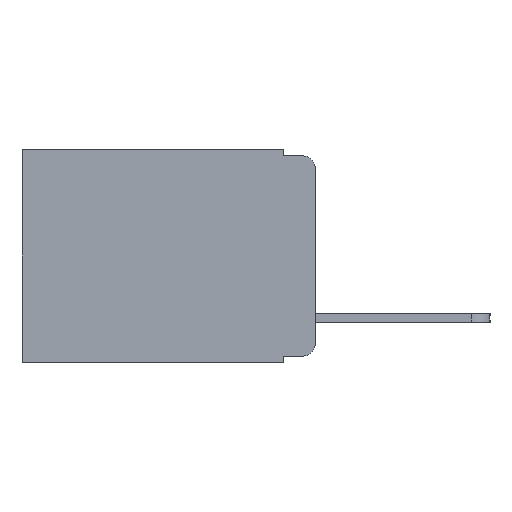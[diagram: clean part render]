
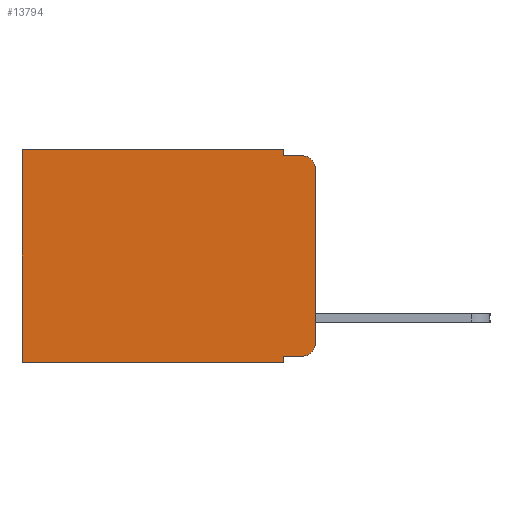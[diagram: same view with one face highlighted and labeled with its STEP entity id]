
A CAD part, left-side view. The second image highlights one B-rep face of the part: STEP entity #13794.
In plain terms, the highlighted planar face has unit normal (-1, 0, 0).
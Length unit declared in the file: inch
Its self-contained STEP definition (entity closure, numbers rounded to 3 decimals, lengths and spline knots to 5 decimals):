
#8 = CIRCLE ( 'NONE', #4290, 0.02 ) ;
#67 = VERTEX_POINT ( 'NONE', #16813 ) ;
#228 = VECTOR ( 'NONE', #5797, 39.37008 ) ;
#309 = CARTESIAN_POINT ( 'NONE',  ( 0.298, 0., -0.313 ) ) ;
#349 = CARTESIAN_POINT ( 'NONE',  ( 0.298, 0.051, 0. ) ) ;
#570 = EDGE_CURVE ( 'NONE', #67, #2575, #5163, .T. ) ;
#610 = LINE ( 'NONE', #349, #3982 ) ;
#619 = DIRECTION ( 'NONE',  ( 0., 0., -1. ) ) ;
#1223 = DIRECTION ( 'NONE',  ( 1., 0., 0. ) ) ;
#1231 = CARTESIAN_POINT ( 'NONE',  ( 0.298, 0.051, -0.343 ) ) ;
#1317 = ORIENTED_EDGE ( 'NONE', *, *, #8128, .T. ) ;
#1391 = VECTOR ( 'NONE', #11471, 39.37008 ) ;
#1469 = CARTESIAN_POINT ( 'NONE',  ( 0.298, 0.051, 0. ) ) ;
#1607 = VECTOR ( 'NONE', #13416, 39.37008 ) ;
#1682 = EDGE_CURVE ( 'NONE', #9458, #18094, #4887, .T. ) ;
#2195 = LINE ( 'NONE', #7707, #13175 ) ;
#2417 = AXIS2_PLACEMENT_3D ( 'NONE', #13843, #5259, #15284 ) ;
#2575 = VERTEX_POINT ( 'NONE', #16688 ) ;
#2893 = ORIENTED_EDGE ( 'NONE', *, *, #8045, .F. ) ;
#2982 = VECTOR ( 'NONE', #619, 39.37008 ) ;
#3013 = VERTEX_POINT ( 'NONE', #4010 ) ;
#3558 = ORIENTED_EDGE ( 'NONE', *, *, #12893, .F. ) ;
#3982 = VECTOR ( 'NONE', #8900, 39.37008 ) ;
#3993 = ORIENTED_EDGE ( 'NONE', *, *, #6020, .T. ) ;
#4010 = CARTESIAN_POINT ( 'NONE',  ( 0.298, 0.02, -0.333 ) ) ;
#4290 = AXIS2_PLACEMENT_3D ( 'NONE', #16778, #8123, #18215 ) ;
#4860 = VERTEX_POINT ( 'NONE', #1231 ) ;
#4887 = LINE ( 'NONE', #9026, #8649 ) ;
#5163 = LINE ( 'NONE', #14113, #9386 ) ;
#5259 = DIRECTION ( 'NONE',  ( -1., 0., 0. ) ) ;
#5569 = ORIENTED_EDGE ( 'NONE', *, *, #6233, .F. ) ;
#5797 = DIRECTION ( 'NONE',  ( 0., 1., 0. ) ) ;
#5806 = CARTESIAN_POINT ( 'NONE',  ( 0.298, 0.051, -0.01 ) ) ;
#6020 = EDGE_CURVE ( 'NONE', #17351, #18094, #8, .T. ) ;
#6233 = EDGE_CURVE ( 'NONE', #4860, #12221, #15062, .T. ) ;
#6262 = CARTESIAN_POINT ( 'NONE',  ( 0.298, 0., -0.03 ) ) ;
#6281 = LINE ( 'NONE', #11976, #1607 ) ;
#7302 = ORIENTED_EDGE ( 'NONE', *, *, #8294, .T. ) ;
#7707 = CARTESIAN_POINT ( 'NONE',  ( 0.298, 0.473, 0. ) ) ;
#8006 = CARTESIAN_POINT ( 'NONE',  ( 0.298, 0.02, -0.01 ) ) ;
#8045 = EDGE_CURVE ( 'NONE', #67, #9458, #610, .T. ) ;
#8123 = DIRECTION ( 'NONE',  ( -1., 0., 0. ) ) ;
#8128 = EDGE_CURVE ( 'NONE', #2575, #12221, #2195, .T. ) ;
#8294 = EDGE_CURVE ( 'NONE', #3013, #14970, #10443, .T. ) ;
#8618 = DIRECTION ( 'NONE',  ( 0., 1., 0. ) ) ;
#8630 = CARTESIAN_POINT ( 'NONE',  ( 0.298, 0., -0.343 ) ) ;
#8649 = VECTOR ( 'NONE', #14306, 39.37008 ) ;
#8660 = VERTEX_POINT ( 'NONE', #18293 ) ;
#8900 = DIRECTION ( 'NONE',  ( 0., 0., -1. ) ) ;
#9026 = CARTESIAN_POINT ( 'NONE',  ( 0.298, 0.051, -0.01 ) ) ;
#9160 = DIRECTION ( 'NONE',  ( 0., 0., -1. ) ) ;
#9386 = VECTOR ( 'NONE', #8618, 39.37008 ) ;
#9458 = VERTEX_POINT ( 'NONE', #5806 ) ;
#10443 = CIRCLE ( 'NONE', #2417, 0.02 ) ;
#10567 = CARTESIAN_POINT ( 'NONE',  ( 0.298, 0.473, -0.343 ) ) ;
#11235 = DIRECTION ( 'NONE',  ( 0., 0., -1. ) ) ;
#11471 = DIRECTION ( 'NONE',  ( 0., 0., -1. ) ) ;
#11976 = CARTESIAN_POINT ( 'NONE',  ( 0.298, 0.051, -0.333 ) ) ;
#12221 = VERTEX_POINT ( 'NONE', #10567 ) ;
#12575 = AXIS2_PLACEMENT_3D ( 'NONE', #15507, #1223, #11235 ) ;
#12893 = EDGE_CURVE ( 'NONE', #17351, #14970, #14860, .T. ) ;
#13175 = VECTOR ( 'NONE', #9160, 39.37008 ) ;
#13416 = DIRECTION ( 'NONE',  ( 0., -1., 0. ) ) ;
#13472 = CARTESIAN_POINT ( 'NONE',  ( 0.298, 0., 0. ) ) ;
#13473 = FACE_OUTER_BOUND ( 'NONE', #15365, .T. ) ;
#13794 = ADVANCED_FACE ( 'NONE', ( #13473 ), #18364, .F. ) ;
#13843 = CARTESIAN_POINT ( 'NONE',  ( 0.298, 0.02, -0.313 ) ) ;
#14113 = CARTESIAN_POINT ( 'NONE',  ( 0.298, 0., 0. ) ) ;
#14306 = DIRECTION ( 'NONE',  ( 0., -1., 0. ) ) ;
#14860 = LINE ( 'NONE', #13472, #2982 ) ;
#14970 = VERTEX_POINT ( 'NONE', #309 ) ;
#15062 = LINE ( 'NONE', #8630, #228 ) ;
#15284 = DIRECTION ( 'NONE',  ( 0., 0., -1. ) ) ;
#15365 = EDGE_LOOP ( 'NONE', ( #3558, #3993, #16316, #2893, #18107, #1317, #5569, #17904, #18338, #7302 ) ) ;
#15507 = CARTESIAN_POINT ( 'NONE',  ( 0.298, 0., 0. ) ) ;
#16316 = ORIENTED_EDGE ( 'NONE', *, *, #1682, .F. ) ;
#16629 = LINE ( 'NONE', #1469, #1391 ) ;
#16688 = CARTESIAN_POINT ( 'NONE',  ( 0.298, 0.473, 0. ) ) ;
#16778 = CARTESIAN_POINT ( 'NONE',  ( 0.298, 0.02, -0.03 ) ) ;
#16813 = CARTESIAN_POINT ( 'NONE',  ( 0.298, 0.051, 0. ) ) ;
#17351 = VERTEX_POINT ( 'NONE', #6262 ) ;
#17726 = EDGE_CURVE ( 'NONE', #8660, #4860, #16629, .T. ) ;
#17904 = ORIENTED_EDGE ( 'NONE', *, *, #17726, .F. ) ;
#17919 = EDGE_CURVE ( 'NONE', #8660, #3013, #6281, .T. ) ;
#18094 = VERTEX_POINT ( 'NONE', #8006 ) ;
#18107 = ORIENTED_EDGE ( 'NONE', *, *, #570, .T. ) ;
#18215 = DIRECTION ( 'NONE',  ( 0., 0., -1. ) ) ;
#18293 = CARTESIAN_POINT ( 'NONE',  ( 0.298, 0.051, -0.333 ) ) ;
#18338 = ORIENTED_EDGE ( 'NONE', *, *, #17919, .T. ) ;
#18364 = PLANE ( 'NONE',  #12575 ) ;
